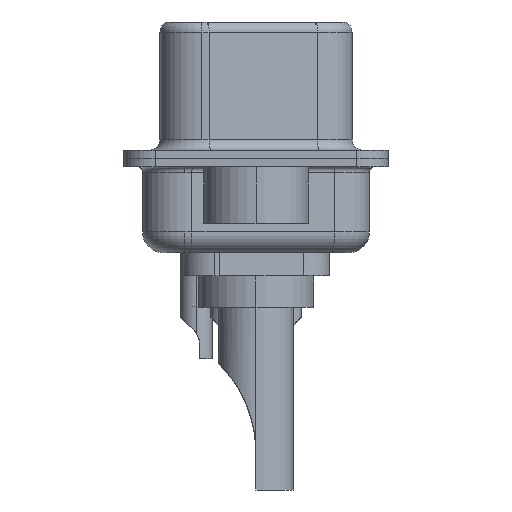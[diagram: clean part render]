
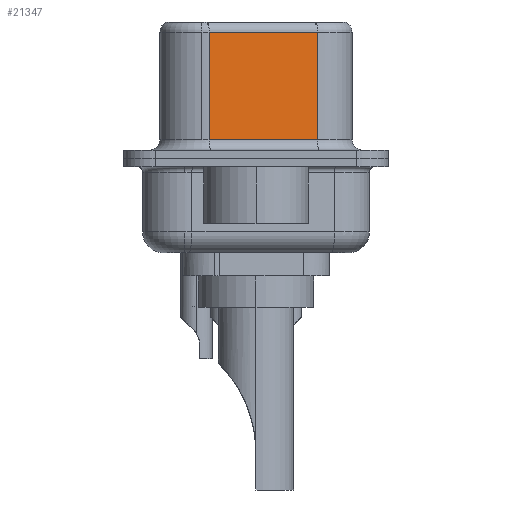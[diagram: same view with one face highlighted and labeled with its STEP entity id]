
A CAD part, left-side view. The second image highlights one B-rep face of the part: STEP entity #21347.
In plain terms, the highlighted planar face has unit normal (-0.985, -0.174, 0).
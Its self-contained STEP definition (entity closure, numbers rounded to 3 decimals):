
#306 = PLANE ( 'NONE',  #10085 ) ;
#2094 = DIRECTION ( 'NONE',  ( 0.985, 0.174, 0. ) ) ;
#2518 = CARTESIAN_POINT ( 'NONE',  ( 4.58, -2.927, 0.9 ) ) ;
#2696 = CARTESIAN_POINT ( 'NONE',  ( 4.58, -2.927, 6.52 ) ) ;
#2862 = CARTESIAN_POINT ( 'NONE',  ( 4.58, -2.927, 6.02 ) ) ;
#3351 = EDGE_LOOP ( 'NONE', ( #15972, #13052, #20973, #13552 ) ) ;
#4761 = VERTEX_POINT ( 'NONE', #8627 ) ;
#5160 = VECTOR ( 'NONE', #16437, 1000. ) ;
#8412 = DIRECTION ( 'NONE',  ( 0., 0., -1. ) ) ;
#8627 = CARTESIAN_POINT ( 'NONE',  ( 3.67, 2.233, 6.02 ) ) ;
#8972 = FACE_OUTER_BOUND ( 'NONE', #3351, .T. ) ;
#9210 = DIRECTION ( 'NONE',  ( 0.174, -0.985, 0. ) ) ;
#9587 = VECTOR ( 'NONE', #9210, 1000. ) ;
#9646 = EDGE_CURVE ( 'NONE', #4761, #19793, #20730, .T. ) ;
#9849 = LINE ( 'NONE', #14598, #5160 ) ;
#10085 = AXIS2_PLACEMENT_3D ( 'NONE', #21942, #2094, #14602 ) ;
#12774 = VERTEX_POINT ( 'NONE', #2862 ) ;
#13052 = ORIENTED_EDGE ( 'NONE', *, *, #20348, .T. ) ;
#13552 = ORIENTED_EDGE ( 'NONE', *, *, #19487, .T. ) ;
#14598 = CARTESIAN_POINT ( 'NONE',  ( 4.58, -2.927, 6.02 ) ) ;
#14602 = DIRECTION ( 'NONE',  ( -0.174, 0.985, 0. ) ) ;
#15172 = CARTESIAN_POINT ( 'NONE',  ( 3.67, 2.233, 0.9 ) ) ;
#15226 = VECTOR ( 'NONE', #8412, 1000. ) ;
#15231 = DIRECTION ( 'NONE',  ( 0., 0., -1. ) ) ;
#15972 = ORIENTED_EDGE ( 'NONE', *, *, #22938, .F. ) ;
#16437 = DIRECTION ( 'NONE',  ( -0.174, 0.985, 0. ) ) ;
#18721 = LINE ( 'NONE', #22004, #9587 ) ;
#19241 = CARTESIAN_POINT ( 'NONE',  ( 3.67, 2.233, 6.52 ) ) ;
#19487 = EDGE_CURVE ( 'NONE', #19793, #19626, #18721, .T. ) ;
#19626 = VERTEX_POINT ( 'NONE', #2518 ) ;
#19793 = VERTEX_POINT ( 'NONE', #15172 ) ;
#20348 = EDGE_CURVE ( 'NONE', #12774, #4761, #9849, .T. ) ;
#20730 = LINE ( 'NONE', #19241, #15226 ) ;
#20973 = ORIENTED_EDGE ( 'NONE', *, *, #9646, .T. ) ;
#21347 = ADVANCED_FACE ( 'NONE', ( #8972 ), #306, .F. ) ;
#21942 = CARTESIAN_POINT ( 'NONE',  ( 4.58, -2.927, 6.52 ) ) ;
#22004 = CARTESIAN_POINT ( 'NONE',  ( 4.58, -2.927, 0.9 ) ) ;
#22077 = VECTOR ( 'NONE', #15231, 1000. ) ;
#22664 = LINE ( 'NONE', #2696, #22077 ) ;
#22938 = EDGE_CURVE ( 'NONE', #12774, #19626, #22664, .T. ) ;
